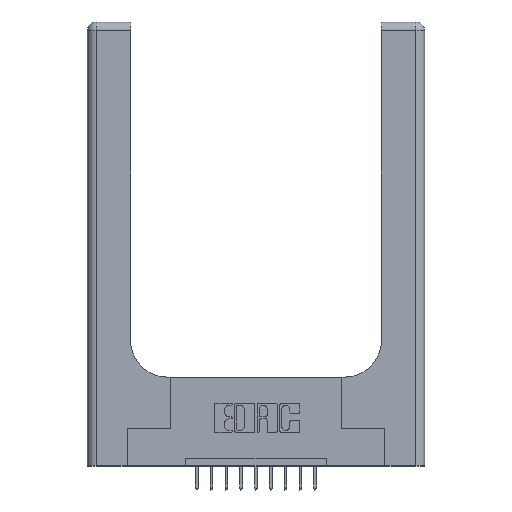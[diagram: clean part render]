
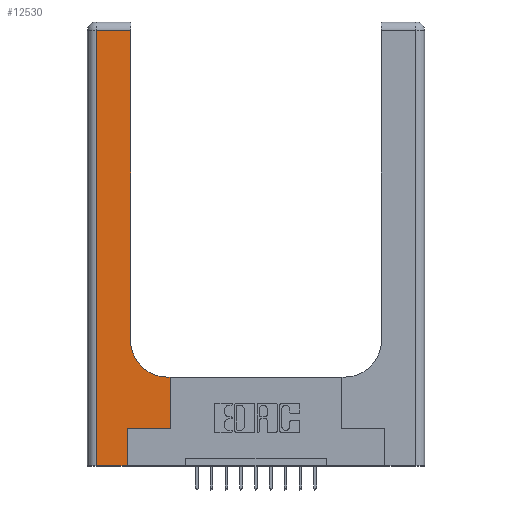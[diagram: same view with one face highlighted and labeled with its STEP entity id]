
A CAD part, top view. The second image highlights one B-rep face of the part: STEP entity #12530.
In plain terms, the highlighted planar face has unit normal (0, 0, 1).
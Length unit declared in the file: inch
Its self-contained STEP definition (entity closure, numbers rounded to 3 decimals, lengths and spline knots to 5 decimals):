
#59 = VECTOR ( 'NONE', #238, 39.37008 ) ;
#230 = VERTEX_POINT ( 'NONE', #6814 ) ;
#238 = DIRECTION ( 'NONE',  ( 0., -1., 0. ) ) ;
#397 = CARTESIAN_POINT ( 'NONE',  ( 0.269, 0., 0.37 ) ) ;
#450 = ORIENTED_EDGE ( 'NONE', *, *, #10103, .T. ) ;
#595 = CARTESIAN_POINT ( 'NONE',  ( 0.5415, 0.85, 0.37 ) ) ;
#839 = VECTOR ( 'NONE', #5912, 39.37008 ) ;
#846 = DIRECTION ( 'NONE',  ( 0., 1., 0. ) ) ;
#849 = CARTESIAN_POINT ( 'NONE',  ( 0.269, 0.25, 0.37 ) ) ;
#1355 = CARTESIAN_POINT ( 'NONE',  ( 0.2915, 0.6, 0.37 ) ) ;
#2224 = CARTESIAN_POINT ( 'NONE',  ( 0.5585, 0.6, 0.37 ) ) ;
#2805 = FACE_OUTER_BOUND ( 'NONE', #9047, .T. ) ;
#3042 = LINE ( 'NONE', #15559, #59 ) ;
#3199 = DIRECTION ( 'NONE',  ( 0., 1., 0. ) ) ;
#3247 = CARTESIAN_POINT ( 'NONE',  ( 0.06, 0., 0.37 ) ) ;
#3802 = CARTESIAN_POINT ( 'NONE',  ( 0.2915, 2.94, 0.37 ) ) ;
#3806 = VERTEX_POINT ( 'NONE', #8603 ) ;
#3954 = PLANE ( 'NONE',  #11414 ) ;
#4130 = DIRECTION ( 'NONE',  ( -1., 0., 0. ) ) ;
#4327 = EDGE_CURVE ( 'NONE', #4519, #15564, #14850, .T. ) ;
#4519 = VERTEX_POINT ( 'NONE', #2224 ) ;
#4795 = CARTESIAN_POINT ( 'NONE',  ( 0.269, 0., 0.37 ) ) ;
#5094 = VECTOR ( 'NONE', #5175, 39.37008 ) ;
#5175 = DIRECTION ( 'NONE',  ( -1., 0., 0. ) ) ;
#5197 = VERTEX_POINT ( 'NONE', #3247 ) ;
#5245 = CARTESIAN_POINT ( 'NONE',  ( 0., 3., 0.37 ) ) ;
#5285 = VECTOR ( 'NONE', #3199, 39.37008 ) ;
#5361 = VECTOR ( 'NONE', #5582, 39.37008 ) ;
#5582 = DIRECTION ( 'NONE',  ( 0., 1., 0. ) ) ;
#5912 = DIRECTION ( 'NONE',  ( 1., 0., 0. ) ) ;
#5927 = ORIENTED_EDGE ( 'NONE', *, *, #6214, .T. ) ;
#6162 = EDGE_CURVE ( 'NONE', #10115, #5197, #3042, .T. ) ;
#6214 = EDGE_CURVE ( 'NONE', #15564, #230, #10650, .T. ) ;
#6288 = EDGE_CURVE ( 'NONE', #5197, #8152, #13224, .T. ) ;
#6561 = EDGE_CURVE ( 'NONE', #12747, #3806, #13393, .T. ) ;
#6814 = CARTESIAN_POINT ( 'NONE',  ( 0.2915, 0.85, 0.37 ) ) ;
#6868 = DIRECTION ( 'NONE',  ( 1., 0., 0. ) ) ;
#7024 = DIRECTION ( 'NONE',  ( 0., 0., -1. ) ) ;
#7548 = ORIENTED_EDGE ( 'NONE', *, *, #15265, .T. ) ;
#7843 = ORIENTED_EDGE ( 'NONE', *, *, #6561, .T. ) ;
#8152 = VERTEX_POINT ( 'NONE', #397 ) ;
#8603 = CARTESIAN_POINT ( 'NONE',  ( 0.5585, 0.25, 0.37 ) ) ;
#8841 = DIRECTION ( 'NONE',  ( -1., 0., 0. ) ) ;
#9047 = EDGE_LOOP ( 'NONE', ( #10903, #450, #14366, #12708, #10545, #7843, #7548, #9418, #5927 ) ) ;
#9087 = DIRECTION ( 'NONE',  ( 0., 0., -1. ) ) ;
#9418 = ORIENTED_EDGE ( 'NONE', *, *, #4327, .T. ) ;
#9452 = VECTOR ( 'NONE', #8841, 39.37008 ) ;
#9563 = DIRECTION ( 'NONE',  ( 1., 0., 0. ) ) ;
#9672 = CARTESIAN_POINT ( 'NONE',  ( 0.5585, 0.25, 0.37 ) ) ;
#10103 = EDGE_CURVE ( 'NONE', #12456, #10115, #12830, .T. ) ;
#10115 = VERTEX_POINT ( 'NONE', #10138 ) ;
#10138 = CARTESIAN_POINT ( 'NONE',  ( 0.06, 2.94, 0.37 ) ) ;
#10545 = ORIENTED_EDGE ( 'NONE', *, *, #11184, .T. ) ;
#10650 = CIRCLE ( 'NONE', #13465, 0.25 ) ;
#10903 = ORIENTED_EDGE ( 'NONE', *, *, #13316, .T. ) ;
#11184 = EDGE_CURVE ( 'NONE', #8152, #12747, #12636, .T. ) ;
#11369 = CARTESIAN_POINT ( 'NONE',  ( 0., 2.94, 0.37 ) ) ;
#11414 = AXIS2_PLACEMENT_3D ( 'NONE', #5245, #9087, #4130 ) ;
#12033 = VECTOR ( 'NONE', #846, 39.37008 ) ;
#12456 = VERTEX_POINT ( 'NONE', #3802 ) ;
#12530 = ADVANCED_FACE ( 'NONE', ( #2805 ), #3954, .F. ) ;
#12636 = LINE ( 'NONE', #4795, #12033 ) ;
#12708 = ORIENTED_EDGE ( 'NONE', *, *, #6288, .T. ) ;
#12747 = VERTEX_POINT ( 'NONE', #13250 ) ;
#12830 = LINE ( 'NONE', #11369, #9452 ) ;
#12957 = LINE ( 'NONE', #13344, #5361 ) ;
#13224 = LINE ( 'NONE', #13453, #16190 ) ;
#13250 = CARTESIAN_POINT ( 'NONE',  ( 0.269, 0.25, 0.37 ) ) ;
#13316 = EDGE_CURVE ( 'NONE', #230, #12456, #12957, .T. ) ;
#13344 = CARTESIAN_POINT ( 'NONE',  ( 0.2915, 3., 0.37 ) ) ;
#13393 = LINE ( 'NONE', #849, #839 ) ;
#13453 = CARTESIAN_POINT ( 'NONE',  ( 0., 0., 0.37 ) ) ;
#13465 = AXIS2_PLACEMENT_3D ( 'NONE', #595, #7024, #6868 ) ;
#13877 = CARTESIAN_POINT ( 'NONE',  ( 0.5415, 0.6, 0.37 ) ) ;
#14075 = LINE ( 'NONE', #9672, #5285 ) ;
#14366 = ORIENTED_EDGE ( 'NONE', *, *, #6162, .T. ) ;
#14850 = LINE ( 'NONE', #1355, #5094 ) ;
#15265 = EDGE_CURVE ( 'NONE', #3806, #4519, #14075, .T. ) ;
#15559 = CARTESIAN_POINT ( 'NONE',  ( 0.06, 3., 0.37 ) ) ;
#15564 = VERTEX_POINT ( 'NONE', #13877 ) ;
#16190 = VECTOR ( 'NONE', #9563, 39.37008 ) ;
